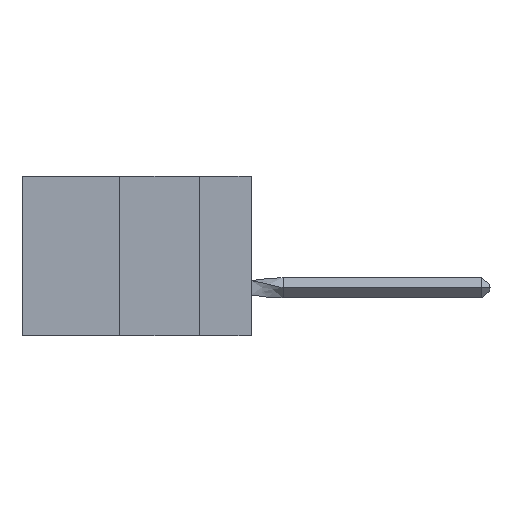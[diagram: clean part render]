
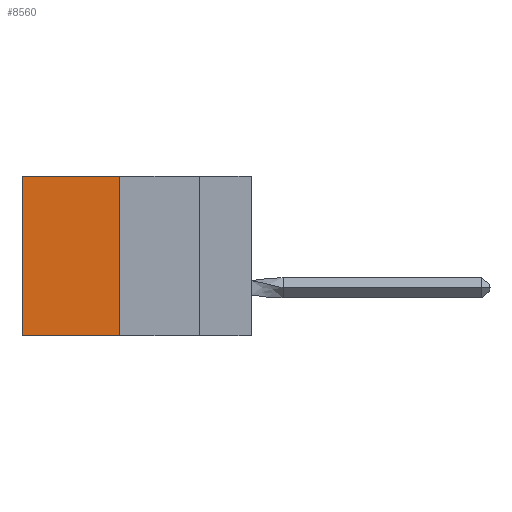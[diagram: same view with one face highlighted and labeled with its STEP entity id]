
A CAD part, left-side view. The second image highlights one B-rep face of the part: STEP entity #8560.
In plain terms, the highlighted planar face has unit normal (-1, 0, 0).
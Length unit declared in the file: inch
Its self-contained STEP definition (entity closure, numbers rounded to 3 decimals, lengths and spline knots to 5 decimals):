
#847 = VERTEX_POINT ( 'NONE', #27771 ) ;
#856 = EDGE_CURVE ( 'NONE', #23062, #21394, #27982, .T. ) ;
#5603 = PLANE ( 'NONE',  #8098 ) ;
#7708 = CARTESIAN_POINT ( 'NONE',  ( 0.305, 0.413, 0. ) ) ;
#8098 = AXIS2_PLACEMENT_3D ( 'NONE', #8317, #23486, #18186 ) ;
#8317 = CARTESIAN_POINT ( 'NONE',  ( 0.305, 0.413, -0.5 ) ) ;
#8560 = ADVANCED_FACE ( 'NONE', ( #10928 ), #5603, .F. ) ;
#9487 = ORIENTED_EDGE ( 'NONE', *, *, #29383, .T. ) ;
#10065 = VECTOR ( 'NONE', #28824, 39.37008 ) ;
#10928 = FACE_OUTER_BOUND ( 'NONE', #11595, .T. ) ;
#11595 = EDGE_LOOP ( 'NONE', ( #25215, #28903, #13165, #9487 ) ) ;
#11886 = LINE ( 'NONE', #7708, #23377 ) ;
#11963 = VECTOR ( 'NONE', #18626, 39.37008 ) ;
#12308 = CARTESIAN_POINT ( 'NONE',  ( 0.305, 0.413, -0.5 ) ) ;
#13165 = ORIENTED_EDGE ( 'NONE', *, *, #22686, .F. ) ;
#13553 = CARTESIAN_POINT ( 'NONE',  ( 0.305, 0.413, -0.5 ) ) ;
#14046 = CARTESIAN_POINT ( 'NONE',  ( 0.305, 0.72, 0. ) ) ;
#14593 = CARTESIAN_POINT ( 'NONE',  ( 0.305, 0.72, -0.5 ) ) ;
#18130 = EDGE_CURVE ( 'NONE', #21090, #21394, #28663, .T. ) ;
#18186 = DIRECTION ( 'NONE',  ( 0., 0., -1. ) ) ;
#18626 = DIRECTION ( 'NONE',  ( 0., 0., -1. ) ) ;
#21090 = VERTEX_POINT ( 'NONE', #14046 ) ;
#21100 = CARTESIAN_POINT ( 'NONE',  ( 0.305, 0.72, -0.5 ) ) ;
#21394 = VERTEX_POINT ( 'NONE', #14593 ) ;
#22686 = EDGE_CURVE ( 'NONE', #847, #23062, #32146, .T. ) ;
#22804 = CARTESIAN_POINT ( 'NONE',  ( 0.305, 0.413, -0.5 ) ) ;
#23062 = VERTEX_POINT ( 'NONE', #22804 ) ;
#23377 = VECTOR ( 'NONE', #29956, 39.37008 ) ;
#23486 = DIRECTION ( 'NONE',  ( 1., 0., 0. ) ) ;
#25215 = ORIENTED_EDGE ( 'NONE', *, *, #18130, .T. ) ;
#27771 = CARTESIAN_POINT ( 'NONE',  ( 0.305, 0.413, 0. ) ) ;
#27982 = LINE ( 'NONE', #12308, #31949 ) ;
#28663 = LINE ( 'NONE', #21100, #10065 ) ;
#28824 = DIRECTION ( 'NONE',  ( 0., 0., -1. ) ) ;
#28903 = ORIENTED_EDGE ( 'NONE', *, *, #856, .F. ) ;
#29383 = EDGE_CURVE ( 'NONE', #847, #21090, #11886, .T. ) ;
#29956 = DIRECTION ( 'NONE',  ( 0., 1., 0. ) ) ;
#30099 = DIRECTION ( 'NONE',  ( 0., 1., 0. ) ) ;
#31949 = VECTOR ( 'NONE', #30099, 39.37008 ) ;
#32146 = LINE ( 'NONE', #13553, #11963 ) ;
